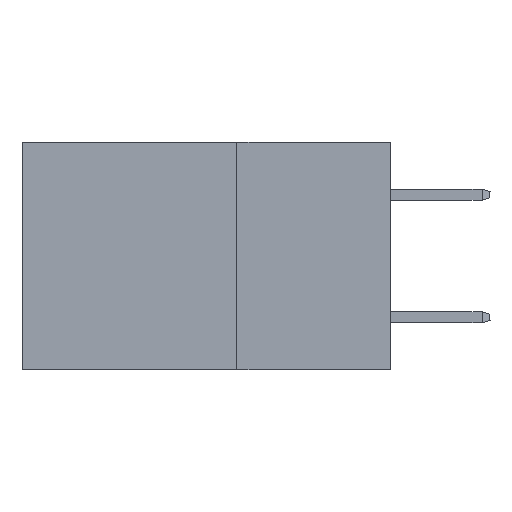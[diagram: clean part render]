
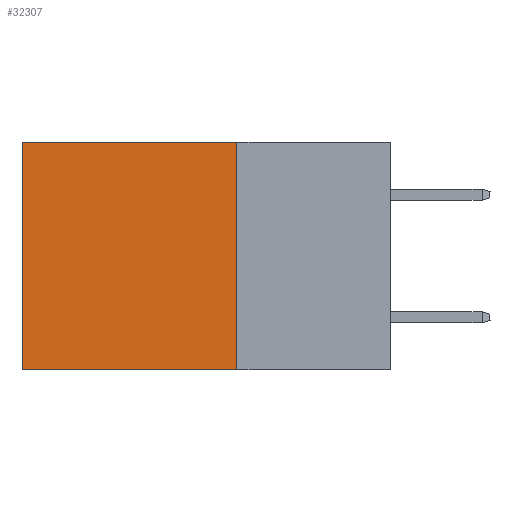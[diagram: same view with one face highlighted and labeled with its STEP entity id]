
A CAD part, left-side view. The second image highlights one B-rep face of the part: STEP entity #32307.
In plain terms, the highlighted planar face has unit normal (-1, 0, 0).
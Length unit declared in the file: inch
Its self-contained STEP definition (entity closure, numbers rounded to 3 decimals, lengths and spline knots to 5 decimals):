
#1169 = DIRECTION ( 'NONE',  ( 1., 0., 0. ) ) ;
#1379 = LINE ( 'NONE', #46878, #7700 ) ;
#2238 = DIRECTION ( 'NONE',  ( 0., 1., 0. ) ) ;
#5053 = DIRECTION ( 'NONE',  ( 0., 0., -1. ) ) ;
#5379 = DIRECTION ( 'NONE',  ( 0., 0., -1. ) ) ;
#6601 = CARTESIAN_POINT ( 'NONE',  ( 0.2875, 0.6, 0. ) ) ;
#7700 = VECTOR ( 'NONE', #2238, 39.37008 ) ;
#8184 = CARTESIAN_POINT ( 'NONE',  ( 0.2875, 0.25, -0.37 ) ) ;
#8330 = LINE ( 'NONE', #31621, #50202 ) ;
#9319 = EDGE_CURVE ( 'NONE', #12652, #31636, #1379, .T. ) ;
#11496 = DIRECTION ( 'NONE',  ( 0., 1., 0. ) ) ;
#12652 = VERTEX_POINT ( 'NONE', #8184 ) ;
#13899 = LINE ( 'NONE', #34282, #39910 ) ;
#14591 = FACE_OUTER_BOUND ( 'NONE', #50672, .T. ) ;
#15443 = AXIS2_PLACEMENT_3D ( 'NONE', #36783, #1169, #5053 ) ;
#18654 = EDGE_CURVE ( 'NONE', #27736, #31636, #8330, .T. ) ;
#19749 = DIRECTION ( 'NONE',  ( 0., 0., -1. ) ) ;
#21736 = CARTESIAN_POINT ( 'NONE',  ( 0.2875, 0.25, 0. ) ) ;
#23629 = ORIENTED_EDGE ( 'NONE', *, *, #47780, .T. ) ;
#24605 = LINE ( 'NONE', #48024, #41069 ) ;
#26673 = ORIENTED_EDGE ( 'NONE', *, *, #9319, .F. ) ;
#27736 = VERTEX_POINT ( 'NONE', #6601 ) ;
#28342 = EDGE_CURVE ( 'NONE', #49881, #12652, #13899, .T. ) ;
#29348 = PLANE ( 'NONE',  #15443 ) ;
#31028 = ORIENTED_EDGE ( 'NONE', *, *, #28342, .F. ) ;
#31621 = CARTESIAN_POINT ( 'NONE',  ( 0.2875, 0.6, 0. ) ) ;
#31636 = VERTEX_POINT ( 'NONE', #33480 ) ;
#32307 = ADVANCED_FACE ( 'NONE', ( #14591 ), #29348, .F. ) ;
#33480 = CARTESIAN_POINT ( 'NONE',  ( 0.2875, 0.6, -0.37 ) ) ;
#34282 = CARTESIAN_POINT ( 'NONE',  ( 0.2875, 0.25, 0. ) ) ;
#36783 = CARTESIAN_POINT ( 'NONE',  ( 0.2875, 0.25, 0. ) ) ;
#39385 = ORIENTED_EDGE ( 'NONE', *, *, #18654, .T. ) ;
#39910 = VECTOR ( 'NONE', #5379, 39.37008 ) ;
#41069 = VECTOR ( 'NONE', #11496, 39.37008 ) ;
#46878 = CARTESIAN_POINT ( 'NONE',  ( 0.2875, 0.25, -0.37 ) ) ;
#47780 = EDGE_CURVE ( 'NONE', #49881, #27736, #24605, .T. ) ;
#48024 = CARTESIAN_POINT ( 'NONE',  ( 0.2875, 0.25, 0. ) ) ;
#49881 = VERTEX_POINT ( 'NONE', #21736 ) ;
#50202 = VECTOR ( 'NONE', #19749, 39.37008 ) ;
#50672 = EDGE_LOOP ( 'NONE', ( #39385, #26673, #31028, #23629 ) ) ;
